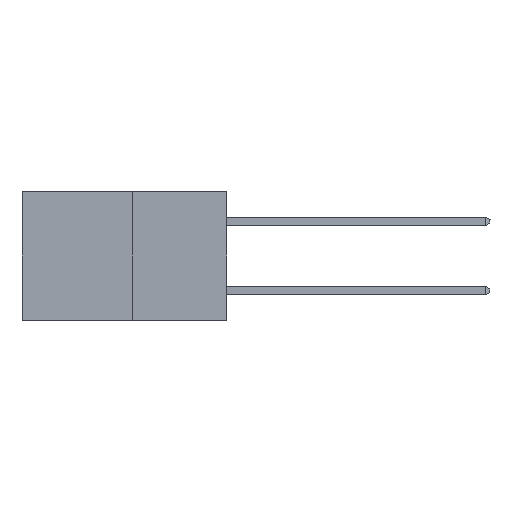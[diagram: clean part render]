
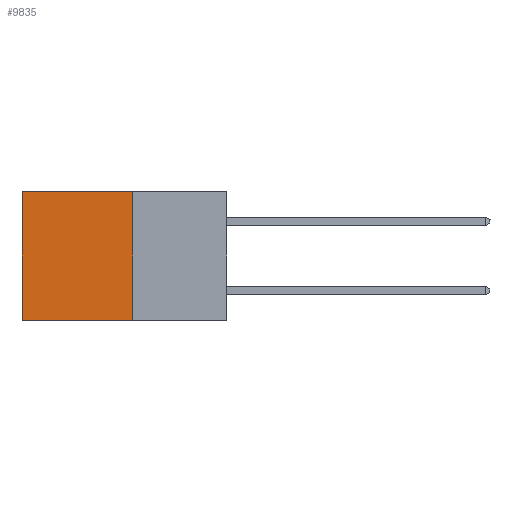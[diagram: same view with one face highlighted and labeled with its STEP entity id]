
A CAD part, left-side view. The second image highlights one B-rep face of the part: STEP entity #9835.
In plain terms, the highlighted planar face has unit normal (-1, 0, 0).
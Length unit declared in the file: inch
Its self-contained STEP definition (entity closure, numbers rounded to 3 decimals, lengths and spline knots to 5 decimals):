
#22 = DIRECTION ( 'NONE',  ( 0., 1., 0. ) ) ;
#223 = VECTOR ( 'NONE', #11197, 39.37008 ) ;
#470 = VECTOR ( 'NONE', #9604, 39.37008 ) ;
#1466 = CARTESIAN_POINT ( 'NONE',  ( 0.277, 0.27, -0.37 ) ) ;
#2197 = CARTESIAN_POINT ( 'NONE',  ( 0.277, 0.27, 0. ) ) ;
#2234 = LINE ( 'NONE', #7405, #2628 ) ;
#2628 = VECTOR ( 'NONE', #22, 39.37008 ) ;
#3777 = ORIENTED_EDGE ( 'NONE', *, *, #15768, .F. ) ;
#3908 = AXIS2_PLACEMENT_3D ( 'NONE', #6966, #15419, #8187 ) ;
#4357 = EDGE_LOOP ( 'NONE', ( #5834, #3777, #8335, #8727 ) ) ;
#5045 = CARTESIAN_POINT ( 'NONE',  ( 0.277, 0.27, 0. ) ) ;
#5264 = VERTEX_POINT ( 'NONE', #9083 ) ;
#5499 = FACE_OUTER_BOUND ( 'NONE', #4357, .T. ) ;
#5834 = ORIENTED_EDGE ( 'NONE', *, *, #8543, .T. ) ;
#6782 = LINE ( 'NONE', #5045, #223 ) ;
#6966 = CARTESIAN_POINT ( 'NONE',  ( 0.277, 0.27, -0.37 ) ) ;
#7405 = CARTESIAN_POINT ( 'NONE',  ( 0.277, 0.27, -0.37 ) ) ;
#7569 = LINE ( 'NONE', #1466, #13682 ) ;
#8187 = DIRECTION ( 'NONE',  ( 0., 0., -1. ) ) ;
#8335 = ORIENTED_EDGE ( 'NONE', *, *, #15023, .F. ) ;
#8543 = EDGE_CURVE ( 'NONE', #9480, #8627, #10291, .T. ) ;
#8627 = VERTEX_POINT ( 'NONE', #10944 ) ;
#8727 = ORIENTED_EDGE ( 'NONE', *, *, #10845, .T. ) ;
#9083 = CARTESIAN_POINT ( 'NONE',  ( 0.277, 0.27, -0.37 ) ) ;
#9480 = VERTEX_POINT ( 'NONE', #10001 ) ;
#9604 = DIRECTION ( 'NONE',  ( 0., 0., -1. ) ) ;
#9835 = ADVANCED_FACE ( 'NONE', ( #5499 ), #14264, .F. ) ;
#10001 = CARTESIAN_POINT ( 'NONE',  ( 0.277, 0.59, 0. ) ) ;
#10291 = LINE ( 'NONE', #15564, #470 ) ;
#10845 = EDGE_CURVE ( 'NONE', #12835, #9480, #6782, .T. ) ;
#10944 = CARTESIAN_POINT ( 'NONE',  ( 0.277, 0.59, -0.37 ) ) ;
#11197 = DIRECTION ( 'NONE',  ( 0., 1., 0. ) ) ;
#12541 = DIRECTION ( 'NONE',  ( 0., 0., -1. ) ) ;
#12835 = VERTEX_POINT ( 'NONE', #2197 ) ;
#13682 = VECTOR ( 'NONE', #12541, 39.37008 ) ;
#14264 = PLANE ( 'NONE',  #3908 ) ;
#15023 = EDGE_CURVE ( 'NONE', #12835, #5264, #7569, .T. ) ;
#15419 = DIRECTION ( 'NONE',  ( 1., 0., 0. ) ) ;
#15564 = CARTESIAN_POINT ( 'NONE',  ( 0.277, 0.59, -0.37 ) ) ;
#15768 = EDGE_CURVE ( 'NONE', #5264, #8627, #2234, .T. ) ;
